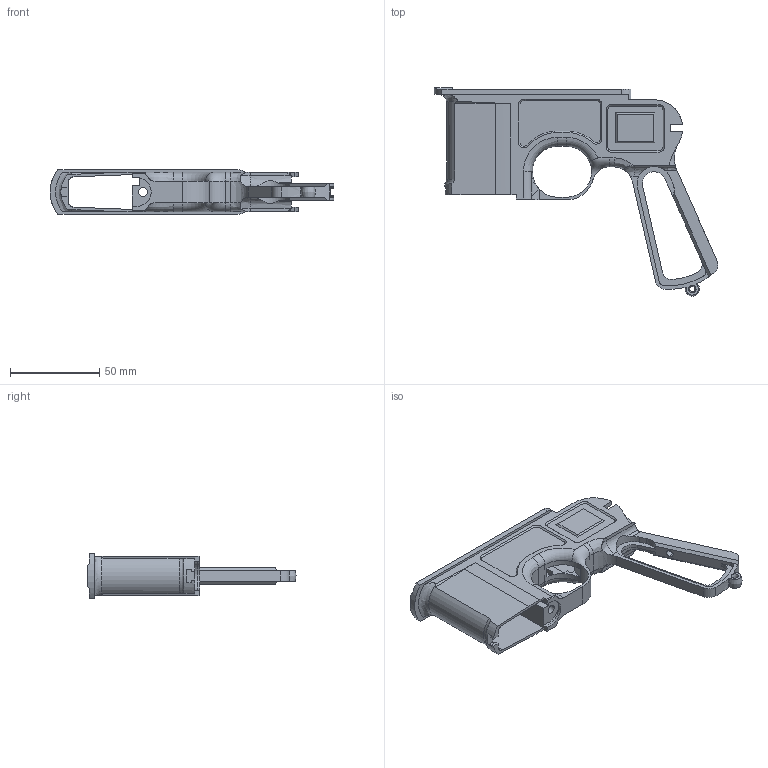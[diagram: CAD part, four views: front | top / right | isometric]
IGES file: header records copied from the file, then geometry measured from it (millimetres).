
Global section: file name: No Iges File Name specified; native system: Autodesk Inventor 2011; preprocessor: AutoDesk Inventor Iges Exporter R2011; author: EfimchenkoPA; date: 20111124.153810; units: millimetre
Bounding box: 158.67 x 116.52 x 25 mm (x, y, z)
Volume: 39561.2 mm3; surface area: 38511.2 mm2
Topology: 1 solids, 1 shells, 351 faces, 1021 edges, 666 vertices
Faces by surface type: plane 166, revolution 101, bspline 56, cylinder 20, torus 4, cone 4
